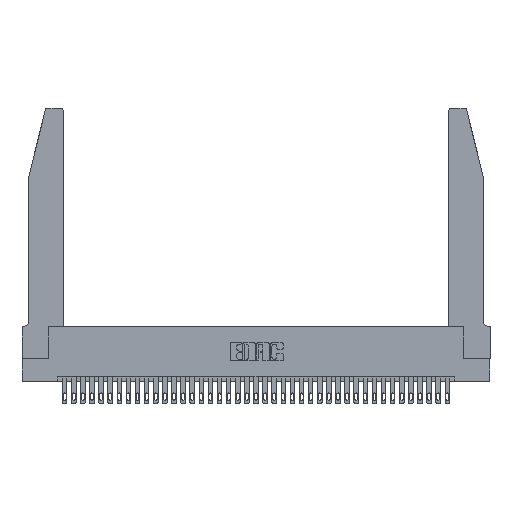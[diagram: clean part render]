
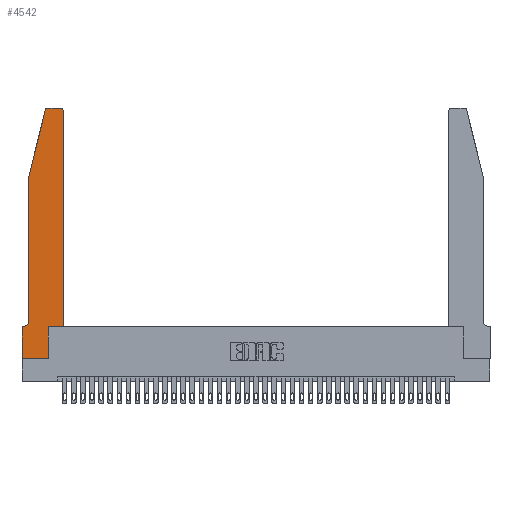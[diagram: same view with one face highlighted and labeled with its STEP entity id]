
A CAD part, top view. The second image highlights one B-rep face of the part: STEP entity #4542.
In plain terms, the highlighted planar face has unit normal (0, 0, 1).
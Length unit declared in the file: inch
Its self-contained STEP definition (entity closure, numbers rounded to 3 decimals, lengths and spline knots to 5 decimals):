
#800 = CARTESIAN_POINT ( 'NONE',  ( 0.0055, 0.42, 0.37 ) ) ;
#1029 = DIRECTION ( 'NONE',  ( -1., 0., 0. ) ) ;
#1682 = ORIENTED_EDGE ( 'NONE', *, *, #31895, .T. ) ;
#2172 = DIRECTION ( 'NONE',  ( 1., 0., 0. ) ) ;
#2222 = DIRECTION ( 'NONE',  ( 0., -1., 0. ) ) ;
#3162 = ORIENTED_EDGE ( 'NONE', *, *, #16168, .T. ) ;
#3421 = CARTESIAN_POINT ( 'NONE',  ( 0.2865, 0.35, 0.37 ) ) ;
#3611 = VERTEX_POINT ( 'NONE', #22242 ) ;
#3927 = DIRECTION ( 'NONE',  ( 1., 0., 0. ) ) ;
#4189 = CARTESIAN_POINT ( 'NONE',  ( 0., 0., 0.37 ) ) ;
#4234 = VECTOR ( 'NONE', #24178, 39.37008 ) ;
#4400 = VERTEX_POINT ( 'NONE', #35806 ) ;
#4542 = ADVANCED_FACE ( 'NONE', ( #36102 ), #7997, .T. ) ;
#4828 = VECTOR ( 'NONE', #6896, 39.37008 ) ;
#4985 = LINE ( 'NONE', #22854, #35138 ) ;
#5010 = CARTESIAN_POINT ( 'NONE',  ( 0., 0., 0.37 ) ) ;
#5101 = CARTESIAN_POINT ( 'NONE',  ( 0., 0.35, 0.37 ) ) ;
#5252 = CIRCLE ( 'NONE', #17142, 0.03 ) ;
#5406 = ORIENTED_EDGE ( 'NONE', *, *, #8388, .T. ) ;
#6402 = CARTESIAN_POINT ( 'NONE',  ( 0.4505, 0.35, 0.37 ) ) ;
#6474 = VERTEX_POINT ( 'NONE', #6772 ) ;
#6772 = CARTESIAN_POINT ( 'NONE',  ( 0.25487, 2.72718, 0.37 ) ) ;
#6896 = DIRECTION ( 'NONE',  ( 1., 0., 0. ) ) ;
#7281 = VERTEX_POINT ( 'NONE', #37628 ) ;
#7391 = ORIENTED_EDGE ( 'NONE', *, *, #15460, .T. ) ;
#7494 = LINE ( 'NONE', #6402, #38098 ) ;
#7894 = ORIENTED_EDGE ( 'NONE', *, *, #34607, .T. ) ;
#7997 = PLANE ( 'NONE',  #27445 ) ;
#8299 = CARTESIAN_POINT ( 'NONE',  ( 0.0755, 2., 0.37 ) ) ;
#8388 = EDGE_CURVE ( 'NONE', #6474, #14553, #33709, .T. ) ;
#8410 = LINE ( 'NONE', #32415, #4234 ) ;
#10448 = EDGE_CURVE ( 'NONE', #4400, #6474, #5252, .T. ) ;
#10896 = LINE ( 'NONE', #4189, #4828 ) ;
#11095 = EDGE_CURVE ( 'NONE', #35086, #11984, #27947, .T. ) ;
#11984 = VERTEX_POINT ( 'NONE', #22253 ) ;
#12983 = VECTOR ( 'NONE', #1029, 39.37008 ) ;
#13083 = DIRECTION ( 'NONE',  ( -1., 0., 0. ) ) ;
#13233 = VECTOR ( 'NONE', #24750, 39.37008 ) ;
#13958 = VERTEX_POINT ( 'NONE', #5101 ) ;
#13971 = CARTESIAN_POINT ( 'NONE',  ( 0.284, 2.72, 0.37 ) ) ;
#14387 = EDGE_CURVE ( 'NONE', #7281, #35086, #8410, .T. ) ;
#14553 = VERTEX_POINT ( 'NONE', #18183 ) ;
#15460 = EDGE_CURVE ( 'NONE', #11984, #4400, #32875, .T. ) ;
#15520 = DIRECTION ( 'NONE',  ( 1., 0., 0. ) ) ;
#15547 = CARTESIAN_POINT ( 'NONE',  ( 0.4205, 2.72, 0.37 ) ) ;
#15619 = ORIENTED_EDGE ( 'NONE', *, *, #15881, .T. ) ;
#15881 = EDGE_CURVE ( 'NONE', #3611, #20474, #30972, .T. ) ;
#16168 = EDGE_CURVE ( 'NONE', #14553, #3611, #4985, .T. ) ;
#17142 = AXIS2_PLACEMENT_3D ( 'NONE', #13971, #37627, #2172 ) ;
#17392 = AXIS2_PLACEMENT_3D ( 'NONE', #800, #27345, #18329 ) ;
#17697 = VECTOR ( 'NONE', #19117, 39.37008 ) ;
#18183 = CARTESIAN_POINT ( 'NONE',  ( 0.0755, 2., 0.37 ) ) ;
#18329 = DIRECTION ( 'NONE',  ( -1., 0., 0. ) ) ;
#18439 = ORIENTED_EDGE ( 'NONE', *, *, #22511, .T. ) ;
#18539 = CARTESIAN_POINT ( 'NONE',  ( 0.0755, 0.35, 0.37 ) ) ;
#19117 = DIRECTION ( 'NONE',  ( 0., 1., 0. ) ) ;
#19320 = CARTESIAN_POINT ( 'NONE',  ( 0.2605, 2.75, 0.37 ) ) ;
#19500 = EDGE_CURVE ( 'NONE', #32558, #7281, #7494, .T. ) ;
#20432 = LINE ( 'NONE', #18539, #12983 ) ;
#20474 = VERTEX_POINT ( 'NONE', #34726 ) ;
#20953 = ORIENTED_EDGE ( 'NONE', *, *, #10448, .T. ) ;
#22242 = CARTESIAN_POINT ( 'NONE',  ( 0.0755, 0.42, 0.37 ) ) ;
#22253 = CARTESIAN_POINT ( 'NONE',  ( 0.4205, 2.75, 0.37 ) ) ;
#22511 = EDGE_CURVE ( 'NONE', #20474, #13958, #20432, .T. ) ;
#22854 = CARTESIAN_POINT ( 'NONE',  ( 0.0755, 2., 0.37 ) ) ;
#23088 = EDGE_CURVE ( 'NONE', #35280, #34194, #10896, .T. ) ;
#23473 = ORIENTED_EDGE ( 'NONE', *, *, #11095, .T. ) ;
#23836 = ORIENTED_EDGE ( 'NONE', *, *, #23088, .T. ) ;
#24178 = DIRECTION ( 'NONE',  ( 0., 1., 0. ) ) ;
#24357 = LINE ( 'NONE', #36338, #13233 ) ;
#24750 = DIRECTION ( 'NONE',  ( 0., -1., 0. ) ) ;
#25577 = LINE ( 'NONE', #31116, #17697 ) ;
#25605 = CARTESIAN_POINT ( 'NONE',  ( 0.2865, 0., 0.37 ) ) ;
#27345 = DIRECTION ( 'NONE',  ( 0., 0., -1. ) ) ;
#27445 = AXIS2_PLACEMENT_3D ( 'NONE', #28735, #28993, #34679 ) ;
#27947 = CIRCLE ( 'NONE', #33536, 0.03 ) ;
#28549 = EDGE_LOOP ( 'NONE', ( #7391, #20953, #5406, #3162, #15619, #18439, #1682, #23836, #7894, #29752, #37742, #23473 ) ) ;
#28735 = CARTESIAN_POINT ( 'NONE',  ( 0., 0.35, 0.37 ) ) ;
#28993 = DIRECTION ( 'NONE',  ( 0., 0., 1. ) ) ;
#29752 = ORIENTED_EDGE ( 'NONE', *, *, #19500, .T. ) ;
#30972 = CIRCLE ( 'NONE', #17392, 0.07 ) ;
#31116 = CARTESIAN_POINT ( 'NONE',  ( 0.2865, 0.35, 0.37 ) ) ;
#31895 = EDGE_CURVE ( 'NONE', #13958, #35280, #24357, .T. ) ;
#32334 = VECTOR ( 'NONE', #37705, 39.37008 ) ;
#32415 = CARTESIAN_POINT ( 'NONE',  ( 0.4505, 0.35, 0.37 ) ) ;
#32558 = VERTEX_POINT ( 'NONE', #3421 ) ;
#32875 = LINE ( 'NONE', #19320, #35166 ) ;
#33039 = CARTESIAN_POINT ( 'NONE',  ( 0.4505, 2.72, 0.37 ) ) ;
#33536 = AXIS2_PLACEMENT_3D ( 'NONE', #15547, #36220, #3927 ) ;
#33709 = LINE ( 'NONE', #8299, #32334 ) ;
#34194 = VERTEX_POINT ( 'NONE', #25605 ) ;
#34607 = EDGE_CURVE ( 'NONE', #34194, #32558, #25577, .T. ) ;
#34679 = DIRECTION ( 'NONE',  ( 1., 0., 0. ) ) ;
#34726 = CARTESIAN_POINT ( 'NONE',  ( 0.0055, 0.35, 0.37 ) ) ;
#35086 = VERTEX_POINT ( 'NONE', #33039 ) ;
#35138 = VECTOR ( 'NONE', #2222, 39.37008 ) ;
#35166 = VECTOR ( 'NONE', #13083, 39.37008 ) ;
#35280 = VERTEX_POINT ( 'NONE', #5010 ) ;
#35806 = CARTESIAN_POINT ( 'NONE',  ( 0.284, 2.75, 0.37 ) ) ;
#36102 = FACE_OUTER_BOUND ( 'NONE', #28549, .T. ) ;
#36220 = DIRECTION ( 'NONE',  ( 0., 0., 1. ) ) ;
#36338 = CARTESIAN_POINT ( 'NONE',  ( 0., 0., 0.37 ) ) ;
#37627 = DIRECTION ( 'NONE',  ( 0., 0., 1. ) ) ;
#37628 = CARTESIAN_POINT ( 'NONE',  ( 0.4505, 0.35, 0.37 ) ) ;
#37705 = DIRECTION ( 'NONE',  ( -0.239, -0.971, 0. ) ) ;
#37742 = ORIENTED_EDGE ( 'NONE', *, *, #14387, .T. ) ;
#38098 = VECTOR ( 'NONE', #15520, 39.37008 ) ;
